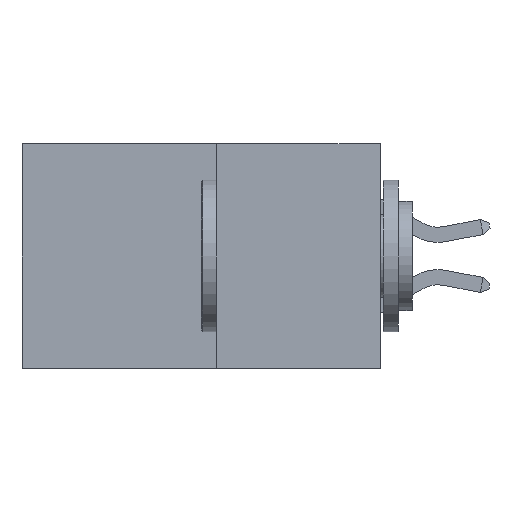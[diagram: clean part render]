
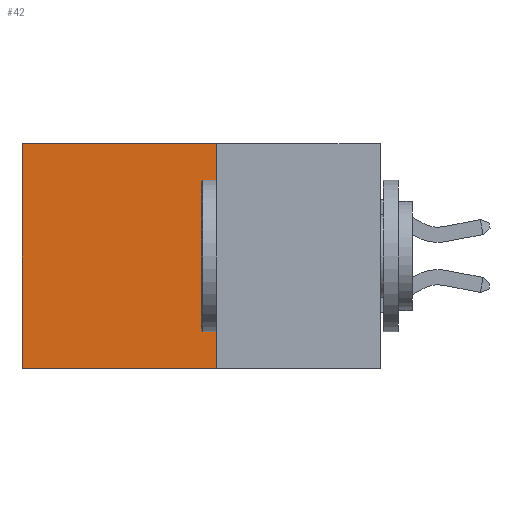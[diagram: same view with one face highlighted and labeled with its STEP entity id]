
A CAD part, left-side view. The second image highlights one B-rep face of the part: STEP entity #42.
In plain terms, the highlighted planar face has unit normal (-1, 0, 0).
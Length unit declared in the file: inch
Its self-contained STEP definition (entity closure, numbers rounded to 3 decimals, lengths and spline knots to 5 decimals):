
#42 = ADVANCED_FACE ( 'NONE', ( #9004 ), #4512, .F. ) ;
#347 = EDGE_LOOP ( 'NONE', ( #10311, #1860, #8486, #10547 ) ) ;
#1197 = VERTEX_POINT ( 'NONE', #6417 ) ;
#1539 = CARTESIAN_POINT ( 'NONE',  ( 0.277, 0.59, -0.37 ) ) ;
#1797 = EDGE_CURVE ( 'NONE', #7292, #1197, #6311, .T. ) ;
#1860 = ORIENTED_EDGE ( 'NONE', *, *, #1797, .F. ) ;
#2305 = VERTEX_POINT ( 'NONE', #7153 ) ;
#2968 = EDGE_CURVE ( 'NONE', #3035, #2305, #9238, .T. ) ;
#3035 = VERTEX_POINT ( 'NONE', #10642 ) ;
#3316 = VECTOR ( 'NONE', #3804, 39.37008 ) ;
#3608 = CARTESIAN_POINT ( 'NONE',  ( 0.277, 0.27, -0.37 ) ) ;
#3804 = DIRECTION ( 'NONE',  ( 0., 0., -1. ) ) ;
#3817 = DIRECTION ( 'NONE',  ( 0., 1., 0. ) ) ;
#4356 = VECTOR ( 'NONE', #3817, 39.37008 ) ;
#4512 = PLANE ( 'NONE',  #6393 ) ;
#4840 = VECTOR ( 'NONE', #7816, 39.37008 ) ;
#5773 = LINE ( 'NONE', #8756, #3316 ) ;
#6311 = LINE ( 'NONE', #3608, #4356 ) ;
#6393 = AXIS2_PLACEMENT_3D ( 'NONE', #7264, #6845, #6416 ) ;
#6416 = DIRECTION ( 'NONE',  ( 0., 0., -1. ) ) ;
#6417 = CARTESIAN_POINT ( 'NONE',  ( 0.277, 0.59, -0.37 ) ) ;
#6834 = LINE ( 'NONE', #1539, #10807 ) ;
#6845 = DIRECTION ( 'NONE',  ( 1., 0., 0. ) ) ;
#7153 = CARTESIAN_POINT ( 'NONE',  ( 0.277, 0.59, 0. ) ) ;
#7264 = CARTESIAN_POINT ( 'NONE',  ( 0.277, 0.27, -0.37 ) ) ;
#7292 = VERTEX_POINT ( 'NONE', #9494 ) ;
#7365 = EDGE_CURVE ( 'NONE', #3035, #7292, #5773, .T. ) ;
#7816 = DIRECTION ( 'NONE',  ( 0., 1., 0. ) ) ;
#8213 = CARTESIAN_POINT ( 'NONE',  ( 0.277, 0.27, 0. ) ) ;
#8372 = EDGE_CURVE ( 'NONE', #2305, #1197, #6834, .T. ) ;
#8486 = ORIENTED_EDGE ( 'NONE', *, *, #7365, .F. ) ;
#8756 = CARTESIAN_POINT ( 'NONE',  ( 0.277, 0.27, -0.37 ) ) ;
#8994 = DIRECTION ( 'NONE',  ( 0., 0., -1. ) ) ;
#9004 = FACE_OUTER_BOUND ( 'NONE', #347, .T. ) ;
#9238 = LINE ( 'NONE', #8213, #4840 ) ;
#9494 = CARTESIAN_POINT ( 'NONE',  ( 0.277, 0.27, -0.37 ) ) ;
#10311 = ORIENTED_EDGE ( 'NONE', *, *, #8372, .T. ) ;
#10547 = ORIENTED_EDGE ( 'NONE', *, *, #2968, .T. ) ;
#10642 = CARTESIAN_POINT ( 'NONE',  ( 0.277, 0.27, 0. ) ) ;
#10807 = VECTOR ( 'NONE', #8994, 39.37008 ) ;
